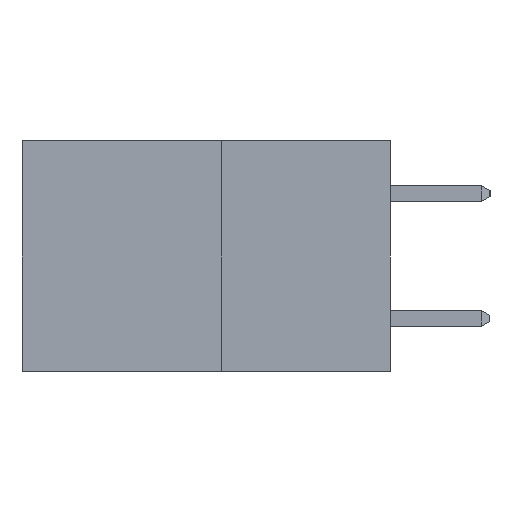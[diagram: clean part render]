
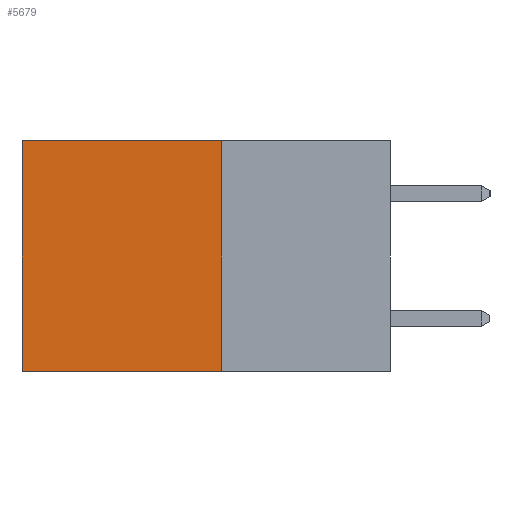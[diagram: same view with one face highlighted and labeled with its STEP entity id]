
A CAD part, left-side view. The second image highlights one B-rep face of the part: STEP entity #5679.
In plain terms, the highlighted planar face has unit normal (-1, 0, 0).
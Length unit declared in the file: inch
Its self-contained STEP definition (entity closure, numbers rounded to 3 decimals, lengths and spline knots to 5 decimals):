
#2236 = LINE ( 'NONE', #5939, #7616 ) ;
#4028 = CARTESIAN_POINT ( 'NONE',  ( 0.277, 0.27, 0. ) ) ;
#5129 = CARTESIAN_POINT ( 'NONE',  ( 0.277, 0.59, 0. ) ) ;
#5381 = DIRECTION ( 'NONE',  ( 0., 1., 0. ) ) ;
#5679 = ADVANCED_FACE ( 'NONE', ( #28872 ), #14215, .F. ) ;
#5939 = CARTESIAN_POINT ( 'NONE',  ( 0.277, 0.27, -0.37 ) ) ;
#6914 = VECTOR ( 'NONE', #15432, 39.37008 ) ;
#7616 = VECTOR ( 'NONE', #5381, 39.37008 ) ;
#8513 = EDGE_CURVE ( 'NONE', #22252, #11190, #2236, .T. ) ;
#9303 = LINE ( 'NONE', #10242, #27516 ) ;
#10034 = VECTOR ( 'NONE', #24686, 39.37008 ) ;
#10242 = CARTESIAN_POINT ( 'NONE',  ( 0.277, 0.59, -0.37 ) ) ;
#10543 = DIRECTION ( 'NONE',  ( 0., 0., -1. ) ) ;
#10691 = ORIENTED_EDGE ( 'NONE', *, *, #8513, .F. ) ;
#11190 = VERTEX_POINT ( 'NONE', #18495 ) ;
#11259 = DIRECTION ( 'NONE',  ( 1., 0., 0. ) ) ;
#14215 = PLANE ( 'NONE',  #16702 ) ;
#14777 = DIRECTION ( 'NONE',  ( 0., 0., -1. ) ) ;
#15432 = DIRECTION ( 'NONE',  ( 0., 0., -1. ) ) ;
#16702 = AXIS2_PLACEMENT_3D ( 'NONE', #17727, #11259, #10543 ) ;
#16718 = EDGE_LOOP ( 'NONE', ( #26336, #10691, #20716, #24655 ) ) ;
#17727 = CARTESIAN_POINT ( 'NONE',  ( 0.277, 0.27, -0.37 ) ) ;
#17986 = CARTESIAN_POINT ( 'NONE',  ( 0.277, 0.27, -0.37 ) ) ;
#18401 = LINE ( 'NONE', #29084, #6914 ) ;
#18495 = CARTESIAN_POINT ( 'NONE',  ( 0.277, 0.59, -0.37 ) ) ;
#20716 = ORIENTED_EDGE ( 'NONE', *, *, #22817, .F. ) ;
#22252 = VERTEX_POINT ( 'NONE', #17986 ) ;
#22486 = VERTEX_POINT ( 'NONE', #5129 ) ;
#22817 = EDGE_CURVE ( 'NONE', #25376, #22252, #18401, .T. ) ;
#23543 = CARTESIAN_POINT ( 'NONE',  ( 0.277, 0.27, 0. ) ) ;
#24655 = ORIENTED_EDGE ( 'NONE', *, *, #28390, .T. ) ;
#24686 = DIRECTION ( 'NONE',  ( 0., 1., 0. ) ) ;
#25376 = VERTEX_POINT ( 'NONE', #23543 ) ;
#26336 = ORIENTED_EDGE ( 'NONE', *, *, #28871, .T. ) ;
#27516 = VECTOR ( 'NONE', #14777, 39.37008 ) ;
#28255 = LINE ( 'NONE', #4028, #10034 ) ;
#28390 = EDGE_CURVE ( 'NONE', #25376, #22486, #28255, .T. ) ;
#28871 = EDGE_CURVE ( 'NONE', #22486, #11190, #9303, .T. ) ;
#28872 = FACE_OUTER_BOUND ( 'NONE', #16718, .T. ) ;
#29084 = CARTESIAN_POINT ( 'NONE',  ( 0.277, 0.27, -0.37 ) ) ;
